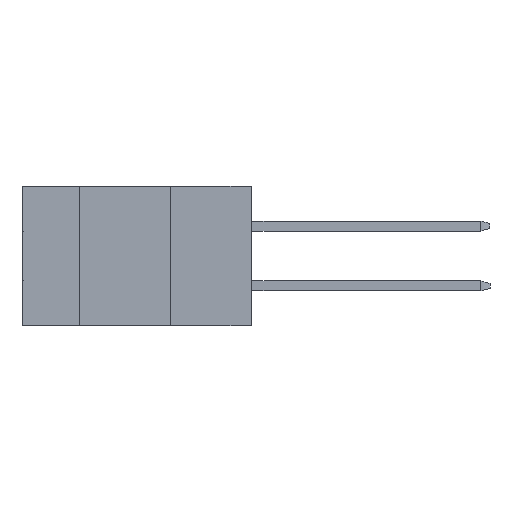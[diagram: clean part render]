
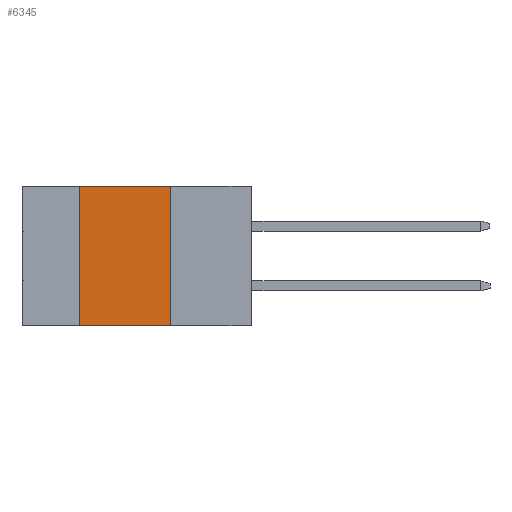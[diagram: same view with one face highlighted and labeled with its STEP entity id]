
A CAD part, left-side view. The second image highlights one B-rep face of the part: STEP entity #6345.
In plain terms, the highlighted planar face has unit normal (-1, 0, 0).
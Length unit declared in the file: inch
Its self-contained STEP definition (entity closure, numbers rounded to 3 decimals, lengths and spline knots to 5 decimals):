
#140 = DIRECTION ( 'NONE',  ( 0., 0., 1. ) ) ;
#629 = AXIS2_PLACEMENT_3D ( 'NONE', #20872, #17261, #3194 ) ;
#805 = ORIENTED_EDGE ( 'NONE', *, *, #14705, .F. ) ;
#2319 = LINE ( 'NONE', #7885, #2383 ) ;
#2383 = VECTOR ( 'NONE', #4317, 39.37008 ) ;
#2992 = EDGE_CURVE ( 'NONE', #9719, #21944, #13957, .T. ) ;
#3194 = DIRECTION ( 'NONE',  ( 0., 0., -1. ) ) ;
#3322 = DIRECTION ( 'NONE',  ( 0., -1., 0. ) ) ;
#4317 = DIRECTION ( 'NONE',  ( 0., -1., 0. ) ) ;
#6345 = ADVANCED_FACE ( 'NONE', ( #22756 ), #19360, .F. ) ;
#7109 = CARTESIAN_POINT ( 'NONE',  ( 0., 0.72, -0.437 ) ) ;
#7864 = LINE ( 'NONE', #11295, #22831 ) ;
#7885 = CARTESIAN_POINT ( 'NONE',  ( 0., 0.72, 0. ) ) ;
#7902 = EDGE_CURVE ( 'NONE', #14880, #21944, #7864, .T. ) ;
#9368 = LINE ( 'NONE', #12895, #22768 ) ;
#9719 = VERTEX_POINT ( 'NONE', #17286 ) ;
#10291 = VECTOR ( 'NONE', #3322, 39.37008 ) ;
#10953 = DIRECTION ( 'NONE',  ( 0., 0., -1. ) ) ;
#10984 = ORIENTED_EDGE ( 'NONE', *, *, #7902, .F. ) ;
#11295 = CARTESIAN_POINT ( 'NONE',  ( 0., 0.254, -0.437 ) ) ;
#12895 = CARTESIAN_POINT ( 'NONE',  ( 0., 0.54, -0.437 ) ) ;
#13928 = ORIENTED_EDGE ( 'NONE', *, *, #20691, .F. ) ;
#13957 = LINE ( 'NONE', #7109, #10291 ) ;
#14603 = EDGE_LOOP ( 'NONE', ( #10984, #13928, #805, #19224 ) ) ;
#14705 = EDGE_CURVE ( 'NONE', #9719, #18177, #9368, .T. ) ;
#14880 = VERTEX_POINT ( 'NONE', #15242 ) ;
#15242 = CARTESIAN_POINT ( 'NONE',  ( 0., 0.254, 0. ) ) ;
#16173 = CARTESIAN_POINT ( 'NONE',  ( 0., 0.54, 0. ) ) ;
#17261 = DIRECTION ( 'NONE',  ( 1., 0., 0. ) ) ;
#17286 = CARTESIAN_POINT ( 'NONE',  ( 0., 0.54, -0.437 ) ) ;
#18177 = VERTEX_POINT ( 'NONE', #16173 ) ;
#19224 = ORIENTED_EDGE ( 'NONE', *, *, #2992, .T. ) ;
#19360 = PLANE ( 'NONE',  #629 ) ;
#20691 = EDGE_CURVE ( 'NONE', #18177, #14880, #2319, .T. ) ;
#20872 = CARTESIAN_POINT ( 'NONE',  ( 0., 0.72, 0. ) ) ;
#21808 = CARTESIAN_POINT ( 'NONE',  ( 0., 0.254, -0.437 ) ) ;
#21944 = VERTEX_POINT ( 'NONE', #21808 ) ;
#22756 = FACE_OUTER_BOUND ( 'NONE', #14603, .T. ) ;
#22768 = VECTOR ( 'NONE', #140, 39.37008 ) ;
#22831 = VECTOR ( 'NONE', #10953, 39.37008 ) ;
